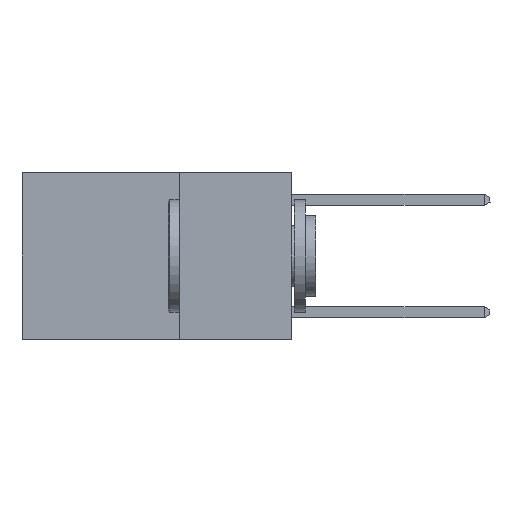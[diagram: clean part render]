
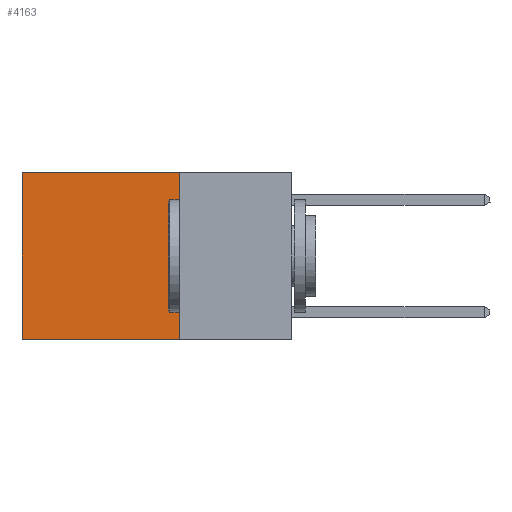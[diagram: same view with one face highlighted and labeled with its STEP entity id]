
A CAD part, left-side view. The second image highlights one B-rep face of the part: STEP entity #4163.
In plain terms, the highlighted planar face has unit normal (-1, 0, 0).
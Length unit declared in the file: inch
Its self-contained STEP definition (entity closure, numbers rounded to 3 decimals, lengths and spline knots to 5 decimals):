
#406 = DIRECTION ( 'NONE',  ( 0., 1., 0. ) ) ;
#464 = EDGE_CURVE ( 'NONE', #11520, #940, #10217, .T. ) ;
#558 = DIRECTION ( 'NONE',  ( 0., 0., -1. ) ) ;
#574 = FACE_OUTER_BOUND ( 'NONE', #5959, .T. ) ;
#706 = DIRECTION ( 'NONE',  ( 0., 0., -1. ) ) ;
#940 = VERTEX_POINT ( 'NONE', #10416 ) ;
#945 = VECTOR ( 'NONE', #8211, 39.37008 ) ;
#1443 = VECTOR ( 'NONE', #406, 39.37008 ) ;
#1617 = ORIENTED_EDGE ( 'NONE', *, *, #8592, .F. ) ;
#1638 = VECTOR ( 'NONE', #706, 39.37008 ) ;
#1886 = CARTESIAN_POINT ( 'NONE',  ( 0.2625, 0.25, 0. ) ) ;
#1927 = LINE ( 'NONE', #11375, #1638 ) ;
#2259 = CARTESIAN_POINT ( 'NONE',  ( 0.2625, 0.25, -0.37 ) ) ;
#2273 = CARTESIAN_POINT ( 'NONE',  ( 0.2625, 0.25, -0.37 ) ) ;
#2604 = PLANE ( 'NONE',  #7860 ) ;
#2642 = CARTESIAN_POINT ( 'NONE',  ( 0.2625, 0.25, 0. ) ) ;
#2999 = VERTEX_POINT ( 'NONE', #2259 ) ;
#3464 = EDGE_CURVE ( 'NONE', #2999, #8279, #8386, .T. ) ;
#4094 = ORIENTED_EDGE ( 'NONE', *, *, #3464, .F. ) ;
#4163 = ADVANCED_FACE ( 'NONE', ( #574 ), #2604, .F. ) ;
#5323 = CARTESIAN_POINT ( 'NONE',  ( 0.2625, 0.25, 0. ) ) ;
#5767 = VECTOR ( 'NONE', #11020, 39.37008 ) ;
#5781 = ORIENTED_EDGE ( 'NONE', *, *, #464, .T. ) ;
#5959 = EDGE_LOOP ( 'NONE', ( #7581, #4094, #1617, #5781 ) ) ;
#7509 = CARTESIAN_POINT ( 'NONE',  ( 0.2625, 0.6, -0.37 ) ) ;
#7566 = EDGE_CURVE ( 'NONE', #940, #8279, #8455, .T. ) ;
#7581 = ORIENTED_EDGE ( 'NONE', *, *, #7566, .T. ) ;
#7860 = AXIS2_PLACEMENT_3D ( 'NONE', #2642, #8561, #558 ) ;
#8211 = DIRECTION ( 'NONE',  ( 0., 1., 0. ) ) ;
#8279 = VERTEX_POINT ( 'NONE', #7509 ) ;
#8386 = LINE ( 'NONE', #2273, #1443 ) ;
#8455 = LINE ( 'NONE', #10695, #5767 ) ;
#8561 = DIRECTION ( 'NONE',  ( 1., 0., 0. ) ) ;
#8592 = EDGE_CURVE ( 'NONE', #11520, #2999, #1927, .T. ) ;
#10217 = LINE ( 'NONE', #1886, #945 ) ;
#10416 = CARTESIAN_POINT ( 'NONE',  ( 0.2625, 0.6, 0. ) ) ;
#10695 = CARTESIAN_POINT ( 'NONE',  ( 0.2625, 0.6, 0. ) ) ;
#11020 = DIRECTION ( 'NONE',  ( 0., 0., -1. ) ) ;
#11375 = CARTESIAN_POINT ( 'NONE',  ( 0.2625, 0.25, 0. ) ) ;
#11520 = VERTEX_POINT ( 'NONE', #5323 ) ;
